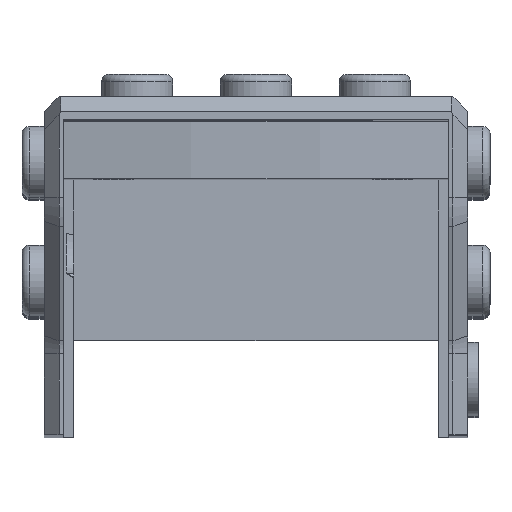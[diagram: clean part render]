
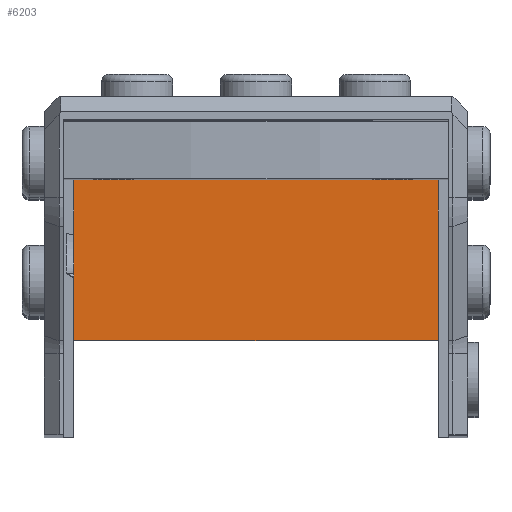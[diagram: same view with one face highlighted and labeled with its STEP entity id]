
A CAD part, top view. The second image highlights one B-rep face of the part: STEP entity #6203.
In plain terms, the highlighted planar face has unit normal (0, 0, 1).
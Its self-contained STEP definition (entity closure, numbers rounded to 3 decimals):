
#541=ORIENTED_EDGE('',*,*,#2147,.F.);
#542=ORIENTED_EDGE('',*,*,#2148,.T.);
#543=ORIENTED_EDGE('',*,*,#2149,.F.);
#544=ORIENTED_EDGE('',*,*,#2150,.F.);
#545=ORIENTED_EDGE('',*,*,#2151,.F.);
#546=ORIENTED_EDGE('',*,*,#2152,.F.);
#2147=EDGE_CURVE('',#2950,#2951,#3565,.T.);
#2148=EDGE_CURVE('',#2950,#2952,#3566,.T.);
#2149=EDGE_CURVE('',#2953,#2952,#3567,.T.);
#2150=EDGE_CURVE('',#2954,#2953,#3568,.T.);
#2151=EDGE_CURVE('',#2955,#2954,#3569,.T.);
#2152=EDGE_CURVE('',#2951,#2955,#3570,.T.);
#2950=VERTEX_POINT('',#9247);
#2951=VERTEX_POINT('',#9248);
#2952=VERTEX_POINT('',#9250);
#2953=VERTEX_POINT('',#9252);
#2954=VERTEX_POINT('',#9254);
#2955=VERTEX_POINT('',#9256);
#3565=LINE('',#9246,#4049);
#3566=LINE('',#9249,#4050);
#3567=LINE('',#9251,#4051);
#3568=LINE('',#9253,#4052);
#3569=LINE('',#9255,#4053);
#3570=LINE('',#9257,#4054);
#4049=VECTOR('',#7372,1000.);
#4050=VECTOR('',#7373,1000.);
#4051=VECTOR('',#7374,1000.);
#4052=VECTOR('',#7375,1000.);
#4053=VECTOR('',#7376,1000.);
#4054=VECTOR('',#7377,1000.);
#4533=EDGE_LOOP('',(#541,#542,#543,#544,#545,#546));
#5245=FACE_BOUND('',#4533,.T.);
#5957=PLANE('',#6673);
#6203=ADVANCED_FACE('',(#5245),#5957,.T.);
#6673=AXIS2_PLACEMENT_3D('',#9245,#7370,#7371);
#7370=DIRECTION('',(0.,0.,1.));
#7371=DIRECTION('',(1.,0.,0.));
#7372=DIRECTION('',(0.,1.,0.));
#7373=DIRECTION('',(1.,0.,0.));
#7374=DIRECTION('',(0.,-1.,0.));
#7375=DIRECTION('',(0.707,-0.707,0.));
#7376=DIRECTION('',(1.,0.,0.));
#7377=DIRECTION('',(0.707,0.707,0.));
#9245=CARTESIAN_POINT('',(0.,0.,-1.));
#9246=CARTESIAN_POINT('',(-12.268,0.254,-1.));
#9247=CARTESIAN_POINT('',(-12.268,6.782,-1.));
#9248=CARTESIAN_POINT('',(-12.268,18.967,-1.));
#9249=CARTESIAN_POINT('',(0.,6.782,-1.));
#9250=CARTESIAN_POINT('',(12.268,6.782,-1.));
#9251=CARTESIAN_POINT('',(12.268,0.254,-1.));
#9252=CARTESIAN_POINT('',(12.268,18.967,-1.));
#9253=CARTESIAN_POINT('',(9.772,21.463,-1.));
#9254=CARTESIAN_POINT('',(9.772,21.463,-1.));
#9255=CARTESIAN_POINT('',(9.772,21.463,-1.));
#9256=CARTESIAN_POINT('',(-9.772,21.463,-1.));
#9257=CARTESIAN_POINT('',(-9.772,21.463,-1.));
